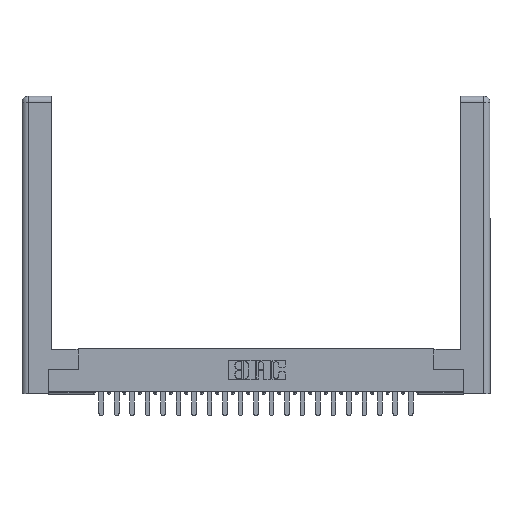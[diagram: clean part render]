
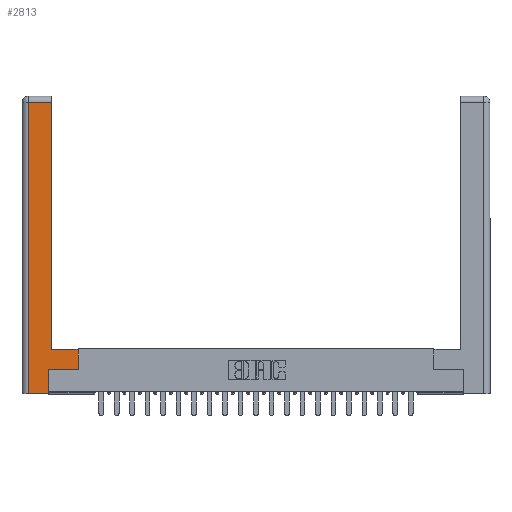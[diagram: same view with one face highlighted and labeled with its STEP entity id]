
A CAD part, top view. The second image highlights one B-rep face of the part: STEP entity #2813.
In plain terms, the highlighted planar face has unit normal (0, 0, 1).
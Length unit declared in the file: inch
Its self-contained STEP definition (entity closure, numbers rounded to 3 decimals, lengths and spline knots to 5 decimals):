
#73 = DIRECTION ( 'NONE',  ( 0., -1., 0. ) ) ;
#167 = EDGE_CURVE ( 'NONE', #4376, #19246, #13783, .T. ) ;
#1199 = LINE ( 'NONE', #7021, #24705 ) ;
#1602 = VERTEX_POINT ( 'NONE', #24356 ) ;
#1616 = VECTOR ( 'NONE', #21053, 39.37008 ) ;
#1856 = ORIENTED_EDGE ( 'NONE', *, *, #4022, .T. ) ;
#2310 = EDGE_CURVE ( 'NONE', #21931, #14977, #5309, .T. ) ;
#2513 = CARTESIAN_POINT ( 'NONE',  ( 0.565, 0.45, 0. ) ) ;
#2813 = ADVANCED_FACE ( 'NONE', ( #21203 ), #9901, .F. ) ;
#3226 = CARTESIAN_POINT ( 'NONE',  ( 0.295, 2.94, 0. ) ) ;
#3509 = LINE ( 'NONE', #7160, #15923 ) ;
#3590 = ORIENTED_EDGE ( 'NONE', *, *, #15560, .T. ) ;
#3889 = VERTEX_POINT ( 'NONE', #3226 ) ;
#4022 = EDGE_CURVE ( 'NONE', #5062, #21931, #19420, .T. ) ;
#4131 = DIRECTION ( 'NONE',  ( 0., 0., -1. ) ) ;
#4235 = DIRECTION ( 'NONE',  ( -1., 0., 0. ) ) ;
#4376 = VERTEX_POINT ( 'NONE', #2513 ) ;
#5062 = VERTEX_POINT ( 'NONE', #11156 ) ;
#5309 = LINE ( 'NONE', #20619, #6028 ) ;
#5402 = DIRECTION ( 'NONE',  ( 1., 0., 0. ) ) ;
#5648 = VECTOR ( 'NONE', #4235, 39.37008 ) ;
#6028 = VECTOR ( 'NONE', #20872, 39.37008 ) ;
#6208 = VECTOR ( 'NONE', #73, 39.37008 ) ;
#7021 = CARTESIAN_POINT ( 'NONE',  ( 0.295, 3., 0. ) ) ;
#7109 = ORIENTED_EDGE ( 'NONE', *, *, #15216, .T. ) ;
#7160 = CARTESIAN_POINT ( 'NONE',  ( 0.265, 0., 0. ) ) ;
#7933 = VECTOR ( 'NONE', #12801, 39.37008 ) ;
#9127 = CARTESIAN_POINT ( 'NONE',  ( 0.0615, 2.94, 0. ) ) ;
#9901 = PLANE ( 'NONE',  #14038 ) ;
#9909 = CARTESIAN_POINT ( 'NONE',  ( 0.295, 0.45, 0. ) ) ;
#10055 = LINE ( 'NONE', #21602, #6208 ) ;
#10923 = VERTEX_POINT ( 'NONE', #18109 ) ;
#11156 = CARTESIAN_POINT ( 'NONE',  ( 0.265, 0., 0. ) ) ;
#11728 = ORIENTED_EDGE ( 'NONE', *, *, #20341, .T. ) ;
#11896 = DIRECTION ( 'NONE',  ( -1., 0., 0. ) ) ;
#12327 = ORIENTED_EDGE ( 'NONE', *, *, #20419, .T. ) ;
#12564 = ORIENTED_EDGE ( 'NONE', *, *, #167, .T. ) ;
#12801 = DIRECTION ( 'NONE',  ( 0., 1., 0. ) ) ;
#13404 = CARTESIAN_POINT ( 'NONE',  ( 0.265, 0.245, 0. ) ) ;
#13783 = LINE ( 'NONE', #21433, #5648 ) ;
#14038 = AXIS2_PLACEMENT_3D ( 'NONE', #24867, #4131, #11896 ) ;
#14815 = CARTESIAN_POINT ( 'NONE',  ( 0.565, 0.45, 0. ) ) ;
#14977 = VERTEX_POINT ( 'NONE', #18327 ) ;
#15216 = EDGE_CURVE ( 'NONE', #19246, #3889, #1199, .T. ) ;
#15560 = EDGE_CURVE ( 'NONE', #10923, #1602, #10055, .T. ) ;
#15923 = VECTOR ( 'NONE', #5402, 39.37008 ) ;
#15938 = ORIENTED_EDGE ( 'NONE', *, *, #2310, .T. ) ;
#16590 = ORIENTED_EDGE ( 'NONE', *, *, #24888, .T. ) ;
#16684 = LINE ( 'NONE', #14815, #7933 ) ;
#17250 = VECTOR ( 'NONE', #18674, 39.37008 ) ;
#18109 = CARTESIAN_POINT ( 'NONE',  ( 0.0615, 2.94, 0. ) ) ;
#18327 = CARTESIAN_POINT ( 'NONE',  ( 0.565, 0.245, 0. ) ) ;
#18674 = DIRECTION ( 'NONE',  ( -1., 0., 0. ) ) ;
#18699 = DIRECTION ( 'NONE',  ( 0., 1., 0. ) ) ;
#18784 = EDGE_LOOP ( 'NONE', ( #7109, #16590, #3590, #11728, #1856, #15938, #12327, #12564 ) ) ;
#19246 = VERTEX_POINT ( 'NONE', #9909 ) ;
#19420 = LINE ( 'NONE', #13404, #1616 ) ;
#20341 = EDGE_CURVE ( 'NONE', #1602, #5062, #3509, .T. ) ;
#20419 = EDGE_CURVE ( 'NONE', #14977, #4376, #16684, .T. ) ;
#20619 = CARTESIAN_POINT ( 'NONE',  ( 0.565, 0.245, 0. ) ) ;
#20872 = DIRECTION ( 'NONE',  ( 1., 0., 0. ) ) ;
#21053 = DIRECTION ( 'NONE',  ( 0., 1., 0. ) ) ;
#21203 = FACE_OUTER_BOUND ( 'NONE', #18784, .T. ) ;
#21433 = CARTESIAN_POINT ( 'NONE',  ( 0.295, 0.45, 0. ) ) ;
#21602 = CARTESIAN_POINT ( 'NONE',  ( 0.0615, 0., 0. ) ) ;
#21931 = VERTEX_POINT ( 'NONE', #23597 ) ;
#23597 = CARTESIAN_POINT ( 'NONE',  ( 0.265, 0.245, 0. ) ) ;
#24204 = LINE ( 'NONE', #9127, #17250 ) ;
#24356 = CARTESIAN_POINT ( 'NONE',  ( 0.0615, 0., 0. ) ) ;
#24705 = VECTOR ( 'NONE', #18699, 39.37008 ) ;
#24867 = CARTESIAN_POINT ( 'NONE',  ( 0., 0., 0. ) ) ;
#24888 = EDGE_CURVE ( 'NONE', #3889, #10923, #24204, .T. ) ;
